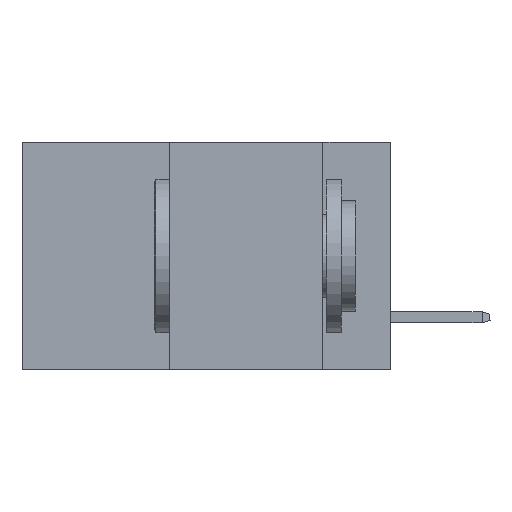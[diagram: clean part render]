
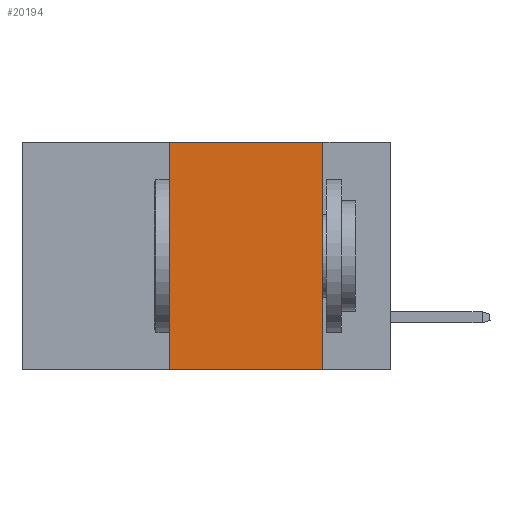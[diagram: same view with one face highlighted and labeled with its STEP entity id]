
A CAD part, left-side view. The second image highlights one B-rep face of the part: STEP entity #20194.
In plain terms, the highlighted planar face has unit normal (-1, 0, 0).
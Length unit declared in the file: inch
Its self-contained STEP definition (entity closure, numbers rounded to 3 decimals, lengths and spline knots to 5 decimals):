
#362 = DIRECTION ( 'NONE',  ( 0., -1., 0. ) ) ;
#1297 = EDGE_CURVE ( 'NONE', #12381, #17636, #24632, .T. ) ;
#2271 = CARTESIAN_POINT ( 'NONE',  ( 0., 0.11, 0. ) ) ;
#3077 = CARTESIAN_POINT ( 'NONE',  ( 0., 0.6, 0. ) ) ;
#4306 = ORIENTED_EDGE ( 'NONE', *, *, #6286, .F. ) ;
#5068 = FACE_OUTER_BOUND ( 'NONE', #9833, .T. ) ;
#5892 = CARTESIAN_POINT ( 'NONE',  ( 0., 0.36, 0. ) ) ;
#6286 = EDGE_CURVE ( 'NONE', #15710, #12381, #21870, .T. ) ;
#7594 = VECTOR ( 'NONE', #362, 39.37008 ) ;
#8867 = DIRECTION ( 'NONE',  ( 0., 0., -1. ) ) ;
#9065 = ORIENTED_EDGE ( 'NONE', *, *, #23169, .F. ) ;
#9833 = EDGE_LOOP ( 'NONE', ( #22819, #4306, #9065, #17570 ) ) ;
#10231 = AXIS2_PLACEMENT_3D ( 'NONE', #3077, #21022, #8867 ) ;
#11091 = DIRECTION ( 'NONE',  ( 0., 0., -1. ) ) ;
#11672 = EDGE_CURVE ( 'NONE', #15358, #17636, #14245, .T. ) ;
#12381 = VERTEX_POINT ( 'NONE', #2271 ) ;
#12752 = VECTOR ( 'NONE', #26071, 39.37008 ) ;
#14176 = CARTESIAN_POINT ( 'NONE',  ( 0., 0.11, -0.37 ) ) ;
#14245 = LINE ( 'NONE', #16365, #7594 ) ;
#15358 = VERTEX_POINT ( 'NONE', #20711 ) ;
#15710 = VERTEX_POINT ( 'NONE', #5892 ) ;
#15906 = CARTESIAN_POINT ( 'NONE',  ( 0., 0.6, 0. ) ) ;
#16365 = CARTESIAN_POINT ( 'NONE',  ( 0., 0.6, -0.37 ) ) ;
#17570 = ORIENTED_EDGE ( 'NONE', *, *, #11672, .T. ) ;
#17636 = VERTEX_POINT ( 'NONE', #14176 ) ;
#18000 = CARTESIAN_POINT ( 'NONE',  ( 0., 0.36, 0. ) ) ;
#18171 = LINE ( 'NONE', #18000, #12752 ) ;
#18964 = PLANE ( 'NONE',  #10231 ) ;
#19230 = VECTOR ( 'NONE', #11091, 39.37008 ) ;
#20194 = ADVANCED_FACE ( 'NONE', ( #5068 ), #18964, .F. ) ;
#20574 = VECTOR ( 'NONE', #25922, 39.37008 ) ;
#20711 = CARTESIAN_POINT ( 'NONE',  ( 0., 0.36, -0.37 ) ) ;
#21022 = DIRECTION ( 'NONE',  ( 1., 0., 0. ) ) ;
#21870 = LINE ( 'NONE', #15906, #20574 ) ;
#22819 = ORIENTED_EDGE ( 'NONE', *, *, #1297, .F. ) ;
#23169 = EDGE_CURVE ( 'NONE', #15358, #15710, #18171, .T. ) ;
#23249 = CARTESIAN_POINT ( 'NONE',  ( 0., 0.11, 0. ) ) ;
#24632 = LINE ( 'NONE', #23249, #19230 ) ;
#25922 = DIRECTION ( 'NONE',  ( 0., -1., 0. ) ) ;
#26071 = DIRECTION ( 'NONE',  ( 0., 0., 1. ) ) ;
